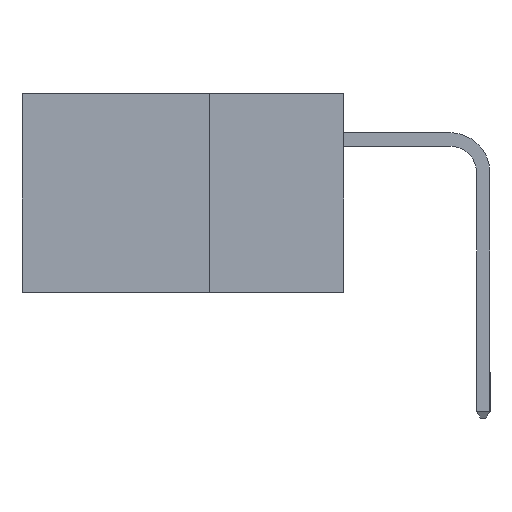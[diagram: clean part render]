
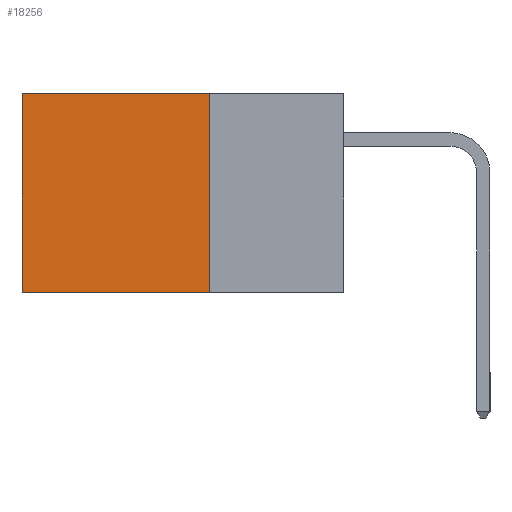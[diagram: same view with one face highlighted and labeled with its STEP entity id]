
A CAD part, left-side view. The second image highlights one B-rep face of the part: STEP entity #18256.
In plain terms, the highlighted planar face has unit normal (-1, 0, 0).
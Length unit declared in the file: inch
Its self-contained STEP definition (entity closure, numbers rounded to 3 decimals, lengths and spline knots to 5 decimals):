
#265 = PLANE ( 'NONE',  #11729 ) ;
#1886 = CARTESIAN_POINT ( 'NONE',  ( 0.298, 0.25, -0.37 ) ) ;
#2160 = CARTESIAN_POINT ( 'NONE',  ( 0.298, 0.25, 0. ) ) ;
#2337 = DIRECTION ( 'NONE',  ( 1., 0., 0. ) ) ;
#3211 = ORIENTED_EDGE ( 'NONE', *, *, #14815, .T. ) ;
#3602 = VERTEX_POINT ( 'NONE', #1886 ) ;
#3772 = LINE ( 'NONE', #20919, #19335 ) ;
#4836 = ORIENTED_EDGE ( 'NONE', *, *, #9378, .F. ) ;
#5694 = VERTEX_POINT ( 'NONE', #11250 ) ;
#5914 = EDGE_CURVE ( 'NONE', #21528, #5694, #22715, .T. ) ;
#5996 = DIRECTION ( 'NONE',  ( 0., 0., -1. ) ) ;
#6840 = LINE ( 'NONE', #2160, #17021 ) ;
#6965 = VECTOR ( 'NONE', #23506, 39.37008 ) ;
#7141 = VECTOR ( 'NONE', #5996, 39.37008 ) ;
#9215 = CARTESIAN_POINT ( 'NONE',  ( 0.298, 0.25, -0.37 ) ) ;
#9378 = EDGE_CURVE ( 'NONE', #3602, #5694, #11742, .T. ) ;
#11250 = CARTESIAN_POINT ( 'NONE',  ( 0.298, 0.6, -0.37 ) ) ;
#11729 = AXIS2_PLACEMENT_3D ( 'NONE', #12506, #2337, #16599 ) ;
#11742 = LINE ( 'NONE', #9215, #6965 ) ;
#12275 = CARTESIAN_POINT ( 'NONE',  ( 0.298, 0.25, 0. ) ) ;
#12506 = CARTESIAN_POINT ( 'NONE',  ( 0.298, 0.25, 0. ) ) ;
#14080 = VERTEX_POINT ( 'NONE', #12275 ) ;
#14815 = EDGE_CURVE ( 'NONE', #14080, #21528, #6840, .T. ) ;
#16422 = DIRECTION ( 'NONE',  ( 0., 1., 0. ) ) ;
#16599 = DIRECTION ( 'NONE',  ( 0., 0., -1. ) ) ;
#16904 = CARTESIAN_POINT ( 'NONE',  ( 0.298, 0.6, 0. ) ) ;
#17021 = VECTOR ( 'NONE', #16422, 39.37008 ) ;
#18198 = CARTESIAN_POINT ( 'NONE',  ( 0.298, 0.6, 0. ) ) ;
#18256 = ADVANCED_FACE ( 'NONE', ( #24828 ), #265, .F. ) ;
#19222 = ORIENTED_EDGE ( 'NONE', *, *, #20967, .F. ) ;
#19335 = VECTOR ( 'NONE', #22945, 39.37008 ) ;
#20919 = CARTESIAN_POINT ( 'NONE',  ( 0.298, 0.25, 0. ) ) ;
#20967 = EDGE_CURVE ( 'NONE', #14080, #3602, #3772, .T. ) ;
#21528 = VERTEX_POINT ( 'NONE', #16904 ) ;
#22715 = LINE ( 'NONE', #18198, #7141 ) ;
#22945 = DIRECTION ( 'NONE',  ( 0., 0., -1. ) ) ;
#23506 = DIRECTION ( 'NONE',  ( 0., 1., 0. ) ) ;
#24695 = ORIENTED_EDGE ( 'NONE', *, *, #5914, .T. ) ;
#24828 = FACE_OUTER_BOUND ( 'NONE', #26180, .T. ) ;
#26180 = EDGE_LOOP ( 'NONE', ( #24695, #4836, #19222, #3211 ) ) ;
